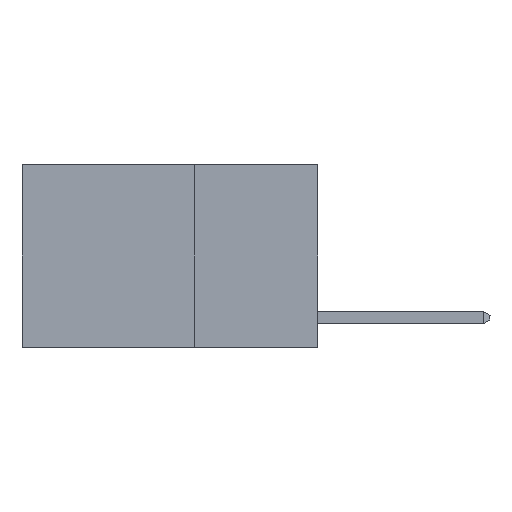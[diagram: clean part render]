
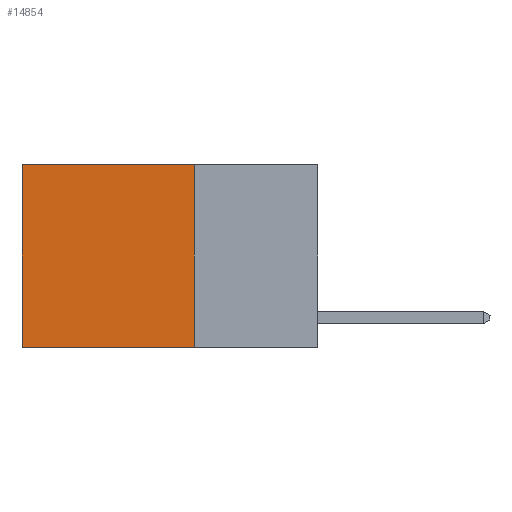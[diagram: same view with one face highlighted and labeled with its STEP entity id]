
A CAD part, left-side view. The second image highlights one B-rep face of the part: STEP entity #14854.
In plain terms, the highlighted planar face has unit normal (-1, 0, 0).
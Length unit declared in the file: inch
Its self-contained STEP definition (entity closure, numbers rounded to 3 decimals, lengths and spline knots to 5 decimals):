
#274 = VERTEX_POINT ( 'NONE', #6480 ) ;
#505 = CARTESIAN_POINT ( 'NONE',  ( 0.2625, 0.25, 0. ) ) ;
#1616 = EDGE_CURVE ( 'NONE', #5678, #12298, #9135, .T. ) ;
#3500 = DIRECTION ( 'NONE',  ( 0., 0., -1. ) ) ;
#3642 = CARTESIAN_POINT ( 'NONE',  ( 0.2625, 0.6, -0.37 ) ) ;
#4630 = LINE ( 'NONE', #18125, #19129 ) ;
#4646 = ORIENTED_EDGE ( 'NONE', *, *, #18529, .F. ) ;
#4882 = DIRECTION ( 'NONE',  ( 0., 1., 0. ) ) ;
#4963 = PLANE ( 'NONE',  #8277 ) ;
#5228 = CARTESIAN_POINT ( 'NONE',  ( 0.2625, 0.25, 0. ) ) ;
#5322 = VECTOR ( 'NONE', #9756, 39.37008 ) ;
#5590 = CARTESIAN_POINT ( 'NONE',  ( 0.2625, 0.25, 0. ) ) ;
#5678 = VERTEX_POINT ( 'NONE', #11378 ) ;
#5914 = EDGE_CURVE ( 'NONE', #10592, #5678, #19092, .T. ) ;
#6480 = CARTESIAN_POINT ( 'NONE',  ( 0.2625, 0.25, -0.37 ) ) ;
#6505 = VECTOR ( 'NONE', #4882, 39.37008 ) ;
#6537 = CARTESIAN_POINT ( 'NONE',  ( 0.2625, 0.25, 0. ) ) ;
#6580 = CARTESIAN_POINT ( 'NONE',  ( 0.2625, 0.6, 0. ) ) ;
#7843 = EDGE_CURVE ( 'NONE', #10592, #274, #17166, .T. ) ;
#8277 = AXIS2_PLACEMENT_3D ( 'NONE', #6537, #10969, #3500 ) ;
#9135 = LINE ( 'NONE', #6580, #16117 ) ;
#9392 = FACE_OUTER_BOUND ( 'NONE', #16352, .T. ) ;
#9756 = DIRECTION ( 'NONE',  ( 0., 0., -1. ) ) ;
#9988 = ORIENTED_EDGE ( 'NONE', *, *, #1616, .T. ) ;
#10258 = ORIENTED_EDGE ( 'NONE', *, *, #5914, .T. ) ;
#10592 = VERTEX_POINT ( 'NONE', #5228 ) ;
#10969 = DIRECTION ( 'NONE',  ( 1., 0., 0. ) ) ;
#11378 = CARTESIAN_POINT ( 'NONE',  ( 0.2625, 0.6, 0. ) ) ;
#11392 = ORIENTED_EDGE ( 'NONE', *, *, #7843, .F. ) ;
#12298 = VERTEX_POINT ( 'NONE', #3642 ) ;
#12884 = DIRECTION ( 'NONE',  ( 0., 1., 0. ) ) ;
#14854 = ADVANCED_FACE ( 'NONE', ( #9392 ), #4963, .F. ) ;
#16117 = VECTOR ( 'NONE', #18320, 39.37008 ) ;
#16352 = EDGE_LOOP ( 'NONE', ( #9988, #4646, #11392, #10258 ) ) ;
#17166 = LINE ( 'NONE', #505, #5322 ) ;
#18125 = CARTESIAN_POINT ( 'NONE',  ( 0.2625, 0.25, -0.37 ) ) ;
#18320 = DIRECTION ( 'NONE',  ( 0., 0., -1. ) ) ;
#18529 = EDGE_CURVE ( 'NONE', #274, #12298, #4630, .T. ) ;
#19092 = LINE ( 'NONE', #5590, #6505 ) ;
#19129 = VECTOR ( 'NONE', #12884, 39.37008 ) ;
